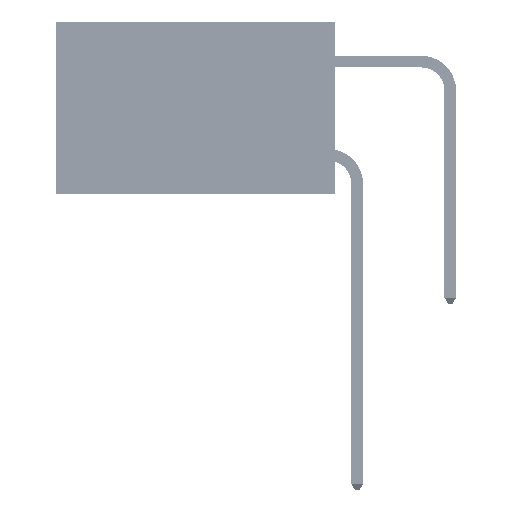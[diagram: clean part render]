
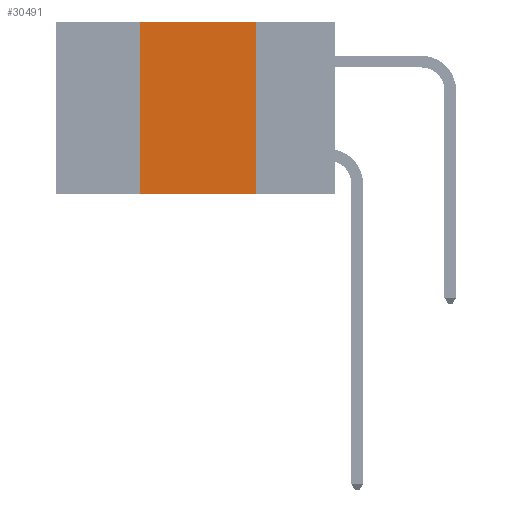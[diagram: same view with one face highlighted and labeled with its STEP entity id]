
A CAD part, left-side view. The second image highlights one B-rep face of the part: STEP entity #30491.
In plain terms, the highlighted planar face has unit normal (-1, 0, 0).
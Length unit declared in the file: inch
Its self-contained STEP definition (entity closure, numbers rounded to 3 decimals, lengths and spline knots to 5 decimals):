
#719 = VERTEX_POINT ( 'NONE', #34213 ) ;
#1395 = CARTESIAN_POINT ( 'NONE',  ( 0., 0.6, -0.37 ) ) ;
#1546 = PLANE ( 'NONE',  #50502 ) ;
#1774 = DIRECTION ( 'NONE',  ( 0., -1., 0. ) ) ;
#4422 = CARTESIAN_POINT ( 'NONE',  ( 0., 0.42, 0. ) ) ;
#5239 = ORIENTED_EDGE ( 'NONE', *, *, #36034, .F. ) ;
#6421 = VERTEX_POINT ( 'NONE', #40917 ) ;
#6558 = VECTOR ( 'NONE', #8461, 39.37008 ) ;
#7169 = DIRECTION ( 'NONE',  ( 0., -1., 0. ) ) ;
#8351 = VECTOR ( 'NONE', #1774, 39.37008 ) ;
#8439 = EDGE_CURVE ( 'NONE', #41087, #36261, #31175, .T. ) ;
#8461 = DIRECTION ( 'NONE',  ( 0., 0., -1. ) ) ;
#9384 = VECTOR ( 'NONE', #7169, 39.37008 ) ;
#10685 = LINE ( 'NONE', #23459, #9384 ) ;
#16868 = CARTESIAN_POINT ( 'NONE',  ( 0., 0.17, 0. ) ) ;
#17489 = EDGE_CURVE ( 'NONE', #719, #6421, #10685, .T. ) ;
#19134 = DIRECTION ( 'NONE',  ( 0., 0., -1. ) ) ;
#21162 = LINE ( 'NONE', #4422, #37991 ) ;
#21834 = DIRECTION ( 'NONE',  ( 0., 0., 1. ) ) ;
#23459 = CARTESIAN_POINT ( 'NONE',  ( 0., 0.6, 0. ) ) ;
#23607 = CARTESIAN_POINT ( 'NONE',  ( 0., 0.6, 0. ) ) ;
#23665 = FACE_OUTER_BOUND ( 'NONE', #45607, .T. ) ;
#27444 = ORIENTED_EDGE ( 'NONE', *, *, #54417, .F. ) ;
#30491 = ADVANCED_FACE ( 'NONE', ( #23665 ), #1546, .F. ) ;
#31175 = LINE ( 'NONE', #1395, #8351 ) ;
#31527 = DIRECTION ( 'NONE',  ( 1., 0., 0. ) ) ;
#34213 = CARTESIAN_POINT ( 'NONE',  ( 0., 0.42, 0. ) ) ;
#35977 = ORIENTED_EDGE ( 'NONE', *, *, #8439, .T. ) ;
#36034 = EDGE_CURVE ( 'NONE', #6421, #36261, #43450, .T. ) ;
#36261 = VERTEX_POINT ( 'NONE', #44241 ) ;
#37991 = VECTOR ( 'NONE', #21834, 39.37008 ) ;
#40917 = CARTESIAN_POINT ( 'NONE',  ( 0., 0.17, 0. ) ) ;
#41087 = VERTEX_POINT ( 'NONE', #47404 ) ;
#43450 = LINE ( 'NONE', #16868, #6558 ) ;
#44241 = CARTESIAN_POINT ( 'NONE',  ( 0., 0.17, -0.37 ) ) ;
#45607 = EDGE_LOOP ( 'NONE', ( #5239, #48500, #27444, #35977 ) ) ;
#47404 = CARTESIAN_POINT ( 'NONE',  ( 0., 0.42, -0.37 ) ) ;
#48500 = ORIENTED_EDGE ( 'NONE', *, *, #17489, .F. ) ;
#50502 = AXIS2_PLACEMENT_3D ( 'NONE', #23607, #31527, #19134 ) ;
#54417 = EDGE_CURVE ( 'NONE', #41087, #719, #21162, .T. ) ;
